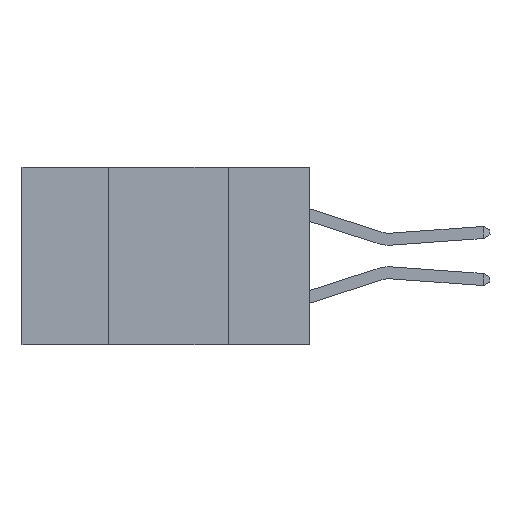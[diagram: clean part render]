
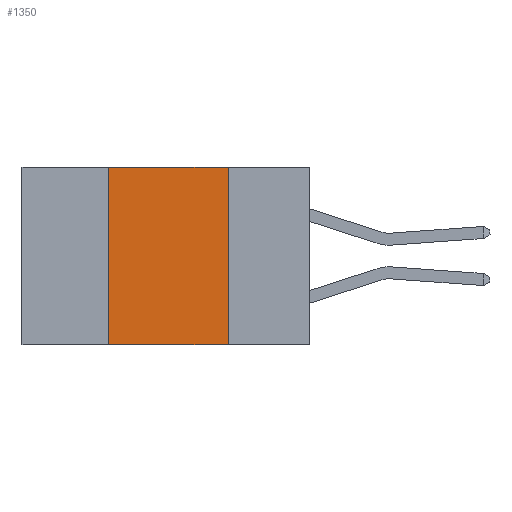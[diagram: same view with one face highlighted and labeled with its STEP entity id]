
A CAD part, left-side view. The second image highlights one B-rep face of the part: STEP entity #1350.
In plain terms, the highlighted planar face has unit normal (-1, 0, 0).
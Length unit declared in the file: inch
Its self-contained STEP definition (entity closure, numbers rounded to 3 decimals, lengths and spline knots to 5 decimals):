
#620 = ORIENTED_EDGE ( 'NONE', *, *, #9352, .F. ) ;
#750 = CARTESIAN_POINT ( 'NONE',  ( 0., 0.6, 0. ) ) ;
#820 = DIRECTION ( 'NONE',  ( 0., -1., 0. ) ) ;
#892 = DIRECTION ( 'NONE',  ( 1., 0., 0. ) ) ;
#1239 = CARTESIAN_POINT ( 'NONE',  ( 0., 0.42, 0. ) ) ;
#1350 = ADVANCED_FACE ( 'NONE', ( #10174 ), #4267, .F. ) ;
#1431 = EDGE_CURVE ( 'NONE', #6905, #4559, #11739, .T. ) ;
#2626 = ORIENTED_EDGE ( 'NONE', *, *, #10014, .T. ) ;
#2946 = CARTESIAN_POINT ( 'NONE',  ( 0., 0.17, -0.37 ) ) ;
#3378 = VECTOR ( 'NONE', #12494, 39.37008 ) ;
#3494 = VECTOR ( 'NONE', #820, 39.37008 ) ;
#3667 = CARTESIAN_POINT ( 'NONE',  ( 0., 0.17, 0. ) ) ;
#3744 = VERTEX_POINT ( 'NONE', #5266 ) ;
#4222 = EDGE_LOOP ( 'NONE', ( #5516, #620, #11978, #2626 ) ) ;
#4267 = PLANE ( 'NONE',  #8882 ) ;
#4435 = DIRECTION ( 'NONE',  ( 0., 0., -1. ) ) ;
#4559 = VERTEX_POINT ( 'NONE', #2946 ) ;
#5266 = CARTESIAN_POINT ( 'NONE',  ( 0., 0.42, -0.37 ) ) ;
#5516 = ORIENTED_EDGE ( 'NONE', *, *, #1431, .F. ) ;
#5952 = LINE ( 'NONE', #8766, #10583 ) ;
#6002 = CARTESIAN_POINT ( 'NONE',  ( 0., 0.42, 0. ) ) ;
#6451 = LINE ( 'NONE', #1239, #3378 ) ;
#6905 = VERTEX_POINT ( 'NONE', #11950 ) ;
#7241 = EDGE_CURVE ( 'NONE', #3744, #7396, #6451, .T. ) ;
#7396 = VERTEX_POINT ( 'NONE', #6002 ) ;
#8336 = CARTESIAN_POINT ( 'NONE',  ( 0., 0.6, 0. ) ) ;
#8473 = LINE ( 'NONE', #750, #3494 ) ;
#8766 = CARTESIAN_POINT ( 'NONE',  ( 0., 0.6, -0.37 ) ) ;
#8882 = AXIS2_PLACEMENT_3D ( 'NONE', #8336, #892, #4435 ) ;
#9352 = EDGE_CURVE ( 'NONE', #7396, #6905, #8473, .T. ) ;
#10001 = DIRECTION ( 'NONE',  ( 0., -1., 0. ) ) ;
#10014 = EDGE_CURVE ( 'NONE', #3744, #4559, #5952, .T. ) ;
#10174 = FACE_OUTER_BOUND ( 'NONE', #4222, .T. ) ;
#10339 = DIRECTION ( 'NONE',  ( 0., 0., -1. ) ) ;
#10583 = VECTOR ( 'NONE', #10001, 39.37008 ) ;
#11475 = VECTOR ( 'NONE', #10339, 39.37008 ) ;
#11739 = LINE ( 'NONE', #3667, #11475 ) ;
#11950 = CARTESIAN_POINT ( 'NONE',  ( 0., 0.17, 0. ) ) ;
#11978 = ORIENTED_EDGE ( 'NONE', *, *, #7241, .F. ) ;
#12494 = DIRECTION ( 'NONE',  ( 0., 0., 1. ) ) ;
